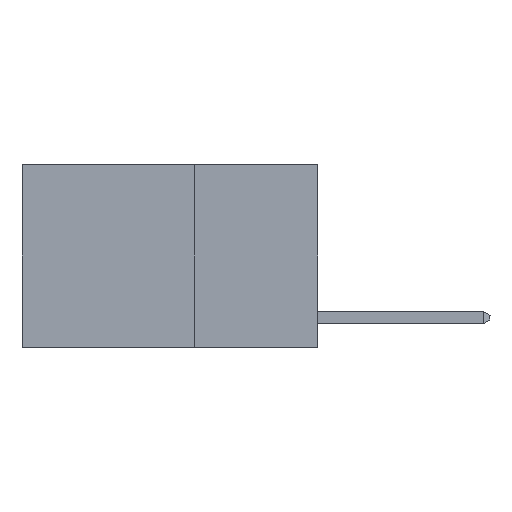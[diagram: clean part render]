
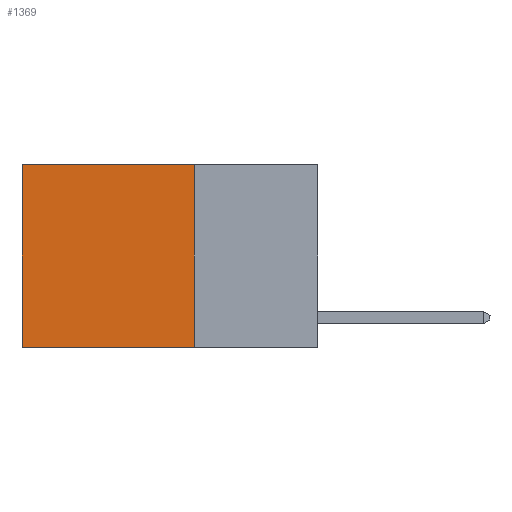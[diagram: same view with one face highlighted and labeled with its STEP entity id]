
A CAD part, left-side view. The second image highlights one B-rep face of the part: STEP entity #1369.
In plain terms, the highlighted planar face has unit normal (-1, 0, 0).
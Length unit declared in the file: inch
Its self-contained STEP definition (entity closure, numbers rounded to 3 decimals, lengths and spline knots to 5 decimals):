
#13 = CARTESIAN_POINT ( 'NONE',  ( 0.2625, 0.25, 0. ) ) ;
#348 = DIRECTION ( 'NONE',  ( 1., 0., 0. ) ) ;
#514 = PLANE ( 'NONE',  #1695 ) ;
#642 = CARTESIAN_POINT ( 'NONE',  ( 0.2625, 0.6, -0.37 ) ) ;
#1369 = ADVANCED_FACE ( 'NONE', ( #4769 ), #514, .F. ) ;
#1624 = VERTEX_POINT ( 'NONE', #10685 ) ;
#1695 = AXIS2_PLACEMENT_3D ( 'NONE', #7333, #348, #10815 ) ;
#2360 = ORIENTED_EDGE ( 'NONE', *, *, #10156, .T. ) ;
#2373 = VECTOR ( 'NONE', #4861, 39.37008 ) ;
#2875 = VERTEX_POINT ( 'NONE', #642 ) ;
#3028 = LINE ( 'NONE', #7434, #4817 ) ;
#3320 = ORIENTED_EDGE ( 'NONE', *, *, #5740, .F. ) ;
#4099 = LINE ( 'NONE', #7599, #10339 ) ;
#4769 = FACE_OUTER_BOUND ( 'NONE', #9830, .T. ) ;
#4817 = VECTOR ( 'NONE', #9079, 39.37008 ) ;
#4861 = DIRECTION ( 'NONE',  ( 0., 1., 0. ) ) ;
#5319 = DIRECTION ( 'NONE',  ( 0., 0., -1. ) ) ;
#5740 = EDGE_CURVE ( 'NONE', #1624, #2875, #11131, .T. ) ;
#6172 = EDGE_CURVE ( 'NONE', #8595, #7227, #4099, .T. ) ;
#7076 = LINE ( 'NONE', #13, #7266 ) ;
#7227 = VERTEX_POINT ( 'NONE', #9762 ) ;
#7266 = VECTOR ( 'NONE', #5319, 39.37008 ) ;
#7333 = CARTESIAN_POINT ( 'NONE',  ( 0.2625, 0.25, 0. ) ) ;
#7434 = CARTESIAN_POINT ( 'NONE',  ( 0.2625, 0.6, 0. ) ) ;
#7599 = CARTESIAN_POINT ( 'NONE',  ( 0.2625, 0.25, 0. ) ) ;
#8595 = VERTEX_POINT ( 'NONE', #10519 ) ;
#9079 = DIRECTION ( 'NONE',  ( 0., 0., -1. ) ) ;
#9340 = ORIENTED_EDGE ( 'NONE', *, *, #10708, .F. ) ;
#9762 = CARTESIAN_POINT ( 'NONE',  ( 0.2625, 0.6, 0. ) ) ;
#9830 = EDGE_LOOP ( 'NONE', ( #2360, #3320, #9340, #9974 ) ) ;
#9974 = ORIENTED_EDGE ( 'NONE', *, *, #6172, .T. ) ;
#10156 = EDGE_CURVE ( 'NONE', #7227, #2875, #3028, .T. ) ;
#10339 = VECTOR ( 'NONE', #11063, 39.37008 ) ;
#10519 = CARTESIAN_POINT ( 'NONE',  ( 0.2625, 0.25, 0. ) ) ;
#10685 = CARTESIAN_POINT ( 'NONE',  ( 0.2625, 0.25, -0.37 ) ) ;
#10708 = EDGE_CURVE ( 'NONE', #8595, #1624, #7076, .T. ) ;
#10815 = DIRECTION ( 'NONE',  ( 0., 0., -1. ) ) ;
#11021 = CARTESIAN_POINT ( 'NONE',  ( 0.2625, 0.25, -0.37 ) ) ;
#11063 = DIRECTION ( 'NONE',  ( 0., 1., 0. ) ) ;
#11131 = LINE ( 'NONE', #11021, #2373 ) ;
